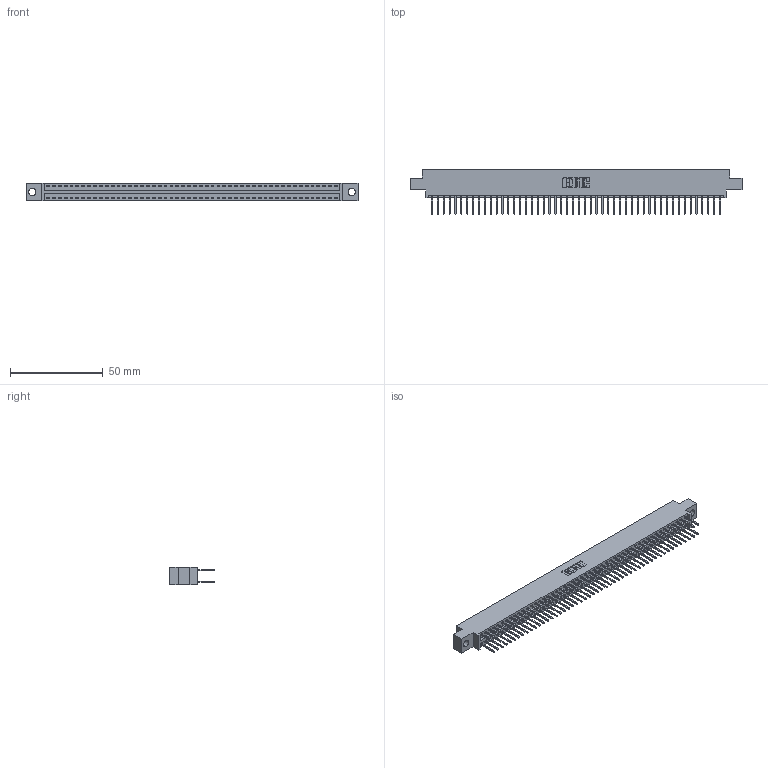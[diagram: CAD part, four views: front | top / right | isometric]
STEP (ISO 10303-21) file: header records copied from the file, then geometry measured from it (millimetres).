
FILE_DESCRIPTION (( 'STEP AP203' ), '1' );
FILE_NAME ('396-100-526-804.STEP', '2018-09-14T07:07:57', ( '' ), ( '' ), 'SwSTEP 2.0', 'SolidWorks 2016', '' );
FILE_SCHEMA (( 'CONFIG_CONTROL_DESIGN' ));
Length unit declared in the file: inch
Products named in the file (3): 346 Part_0.170 Offset - 0.156 Dia-TH; 345-292-001_345-293-126; 396-100-526-804
Assembly tree (101 placements, depth 2):
  396-100-526-804
    346 Part_0.170 Offset - 0.156 Dia-TH
    345-292-001_345-293-126  x100
Bounding box: 179.32 x 24.13 x 9.4 mm (x, y, z)
Volume: 17470 mm3; surface area: 24866.3 mm2
Topology: 101 solids, 101 shells, 5326 faces, 15841 edges, 10426 vertices
Faces by surface type: plane 3580, cylinder 1746
Entity records: 31707 total; most frequent: CARTESIAN_POINT 5216, ORIENTED_EDGE 5150, DIRECTION 4647, EDGE_CURVE 2575, VECTOR 2243, LINE 2243, VERTEX_POINT 1714, AXIS2_PLACEMENT_3D 1202
